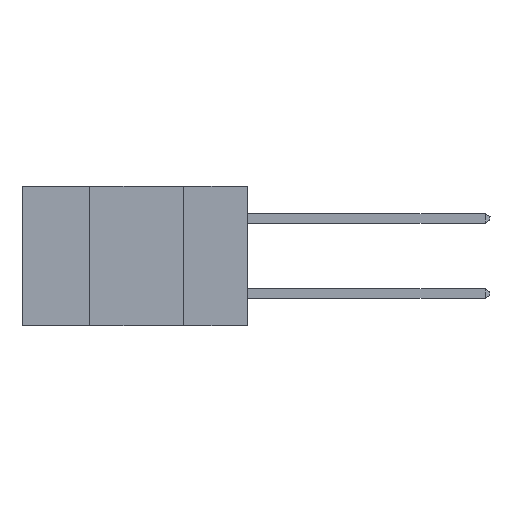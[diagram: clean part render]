
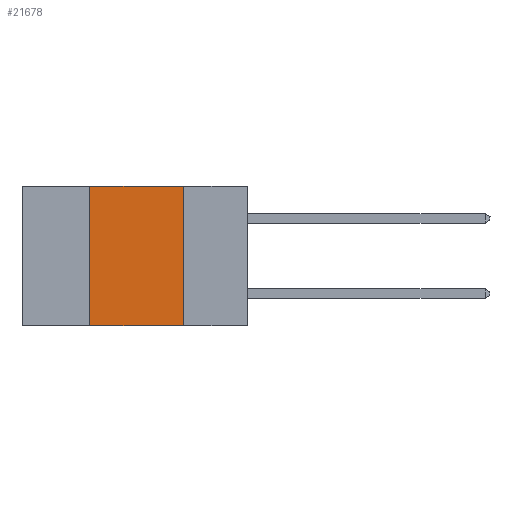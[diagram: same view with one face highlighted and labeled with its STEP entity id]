
A CAD part, left-side view. The second image highlights one B-rep face of the part: STEP entity #21678.
In plain terms, the highlighted planar face has unit normal (-1, 0, 0).
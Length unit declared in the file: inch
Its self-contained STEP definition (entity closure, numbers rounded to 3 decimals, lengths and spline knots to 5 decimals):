
#1609 = DIRECTION ( 'NONE',  ( 1., 0., 0. ) ) ;
#2106 = CARTESIAN_POINT ( 'NONE',  ( 0., 0.42, 0. ) ) ;
#2886 = VERTEX_POINT ( 'NONE', #2106 ) ;
#3535 = FACE_OUTER_BOUND ( 'NONE', #14419, .T. ) ;
#4095 = EDGE_CURVE ( 'NONE', #21135, #15304, #10717, .T. ) ;
#4182 = VECTOR ( 'NONE', #11848, 39.37008 ) ;
#4519 = DIRECTION ( 'NONE',  ( 0., 0., 1. ) ) ;
#5175 = DIRECTION ( 'NONE',  ( 0., 0., -1. ) ) ;
#5535 = ORIENTED_EDGE ( 'NONE', *, *, #4095, .T. ) ;
#5712 = CARTESIAN_POINT ( 'NONE',  ( 0., 0.6, 0. ) ) ;
#7113 = DIRECTION ( 'NONE',  ( 0., -1., 0. ) ) ;
#8285 = VECTOR ( 'NONE', #5175, 39.37008 ) ;
#10692 = ORIENTED_EDGE ( 'NONE', *, *, #16540, .F. ) ;
#10717 = LINE ( 'NONE', #14800, #12446 ) ;
#10801 = CARTESIAN_POINT ( 'NONE',  ( 0., 0.17, -0.37 ) ) ;
#10944 = CARTESIAN_POINT ( 'NONE',  ( 0., 0.17, -0.37 ) ) ;
#11848 = DIRECTION ( 'NONE',  ( 0., -1., 0. ) ) ;
#12446 = VECTOR ( 'NONE', #7113, 39.37008 ) ;
#12672 = ORIENTED_EDGE ( 'NONE', *, *, #20462, .F. ) ;
#14006 = LINE ( 'NONE', #24249, #24014 ) ;
#14419 = EDGE_LOOP ( 'NONE', ( #16125, #10692, #12672, #5535 ) ) ;
#14800 = CARTESIAN_POINT ( 'NONE',  ( 0., 0.6, -0.37 ) ) ;
#15304 = VERTEX_POINT ( 'NONE', #10801 ) ;
#15464 = CARTESIAN_POINT ( 'NONE',  ( 0., 0.17, 0. ) ) ;
#16125 = ORIENTED_EDGE ( 'NONE', *, *, #18742, .F. ) ;
#16540 = EDGE_CURVE ( 'NONE', #2886, #22407, #17728, .T. ) ;
#17516 = AXIS2_PLACEMENT_3D ( 'NONE', #5712, #1609, #19803 ) ;
#17728 = LINE ( 'NONE', #18099, #4182 ) ;
#18099 = CARTESIAN_POINT ( 'NONE',  ( 0., 0.6, 0. ) ) ;
#18742 = EDGE_CURVE ( 'NONE', #22407, #15304, #20426, .T. ) ;
#19803 = DIRECTION ( 'NONE',  ( 0., 0., -1. ) ) ;
#20426 = LINE ( 'NONE', #10944, #8285 ) ;
#20462 = EDGE_CURVE ( 'NONE', #21135, #2886, #14006, .T. ) ;
#21135 = VERTEX_POINT ( 'NONE', #23156 ) ;
#21678 = ADVANCED_FACE ( 'NONE', ( #3535 ), #24930, .F. ) ;
#22407 = VERTEX_POINT ( 'NONE', #15464 ) ;
#23156 = CARTESIAN_POINT ( 'NONE',  ( 0., 0.42, -0.37 ) ) ;
#24014 = VECTOR ( 'NONE', #4519, 39.37008 ) ;
#24249 = CARTESIAN_POINT ( 'NONE',  ( 0., 0.42, -0.37 ) ) ;
#24930 = PLANE ( 'NONE',  #17516 ) ;
